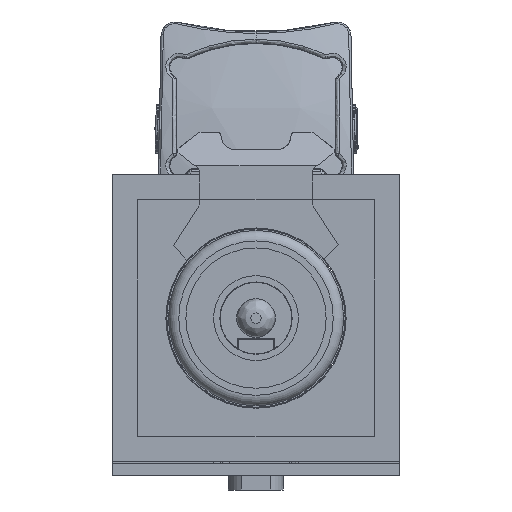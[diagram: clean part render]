
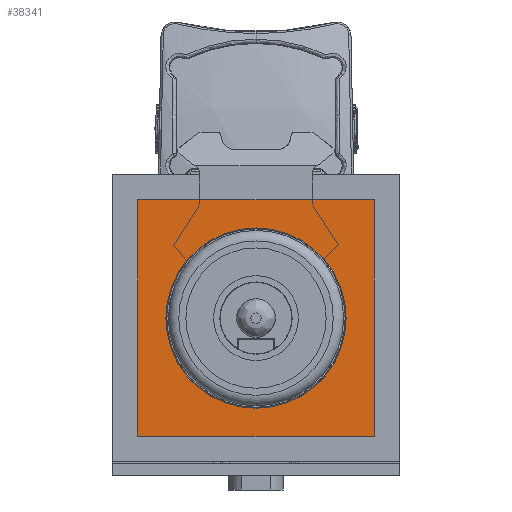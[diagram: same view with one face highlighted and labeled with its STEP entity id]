
A CAD part, front view. The second image highlights one B-rep face of the part: STEP entity #38341.
In plain terms, the highlighted planar face has unit normal (0, -1, 0).
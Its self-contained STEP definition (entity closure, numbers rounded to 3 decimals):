
#408=FACE_BOUND('',#7750,.T.);
#5440=FACE_OUTER_BOUND('',#7749,.T.);
#7749=EDGE_LOOP('',(#35178,#35179,#35180,#35181));
#7750=EDGE_LOOP('',(#35182));
#10595=LINE('',#98765,#13449);
#10596=LINE('',#98767,#13450);
#10597=LINE('',#98769,#13451);
#10598=LINE('',#98770,#13452);
#13449=VECTOR('',#49934,10.);
#13450=VECTOR('',#49935,10.);
#13451=VECTOR('',#49936,10.);
#13452=VECTOR('',#49937,10.);
#14506=CIRCLE('',#41326,12.85);
#18171=VERTEX_POINT('',#98763);
#18172=VERTEX_POINT('',#98764);
#18173=VERTEX_POINT('',#98766);
#18174=VERTEX_POINT('',#98768);
#18175=VERTEX_POINT('',#98771);
#23851=EDGE_CURVE('',#18171,#18172,#10595,.T.);
#23852=EDGE_CURVE('',#18172,#18173,#10596,.T.);
#23853=EDGE_CURVE('',#18173,#18174,#10597,.T.);
#23854=EDGE_CURVE('',#18174,#18171,#10598,.T.);
#23855=EDGE_CURVE('',#18175,#18175,#14506,.T.);
#35178=ORIENTED_EDGE('',*,*,#23851,.T.);
#35179=ORIENTED_EDGE('',*,*,#23852,.T.);
#35180=ORIENTED_EDGE('',*,*,#23853,.T.);
#35181=ORIENTED_EDGE('',*,*,#23854,.T.);
#35182=ORIENTED_EDGE('',*,*,#23855,.T.);
#36223=PLANE('',#41325);
#38341=ADVANCED_FACE('',(#5440,#408),#36223,.F.);
#41325=AXIS2_PLACEMENT_3D('',#98762,#49932,#49933);
#41326=AXIS2_PLACEMENT_3D('',#98772,#49938,#49939);
#49932=DIRECTION('center_axis',(0.,1.,0.));
#49933=DIRECTION('ref_axis',(-1.,0.,0.));
#49934=DIRECTION('',(1.,0.,0.));
#49935=DIRECTION('',(0.,0.,1.));
#49936=DIRECTION('',(-1.,0.,0.));
#49937=DIRECTION('',(0.,0.,-1.));
#49938=DIRECTION('center_axis',(0.,1.,0.));
#49939=DIRECTION('ref_axis',(-1.,0.,0.));
#98762=CARTESIAN_POINT('Origin',(0.,-397.871,
77.687));
#98763=CARTESIAN_POINT('',(-16.859,-397.871,60.828));
#98764=CARTESIAN_POINT('',(16.859,-397.871,60.828));
#98765=CARTESIAN_POINT('',(0.,-397.871,60.828));
#98766=CARTESIAN_POINT('',(16.859,-397.871,94.546));
#98767=CARTESIAN_POINT('',(16.859,-397.871,94.546));
#98768=CARTESIAN_POINT('',(-16.859,-397.871,94.546));
#98769=CARTESIAN_POINT('',(-16.859,-397.871,94.546));
#98770=CARTESIAN_POINT('',(-16.859,-397.871,60.828));
#98771=CARTESIAN_POINT('',(12.85,-397.871,77.687));
#98772=CARTESIAN_POINT('Origin',(0.,-397.871,
77.687));
